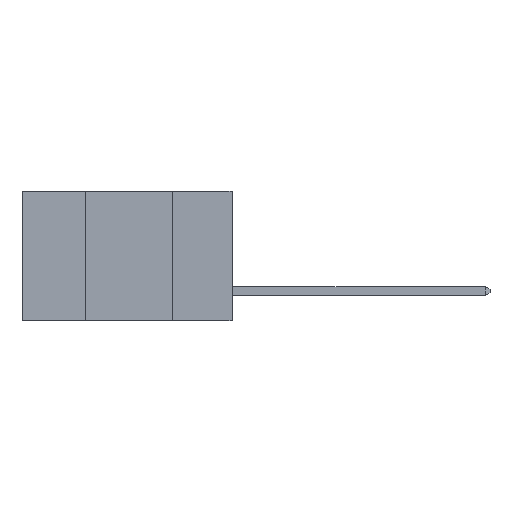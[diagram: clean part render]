
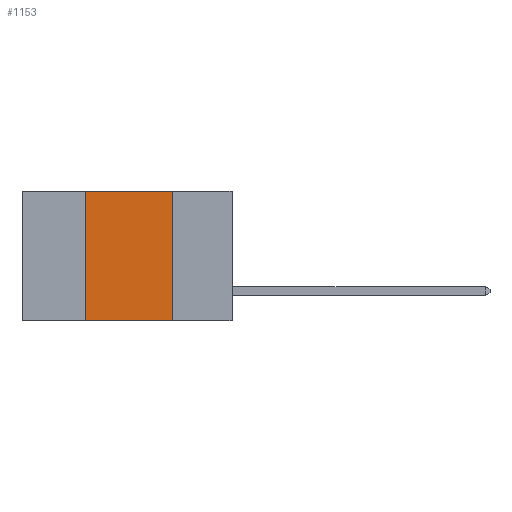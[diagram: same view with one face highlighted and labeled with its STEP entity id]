
A CAD part, left-side view. The second image highlights one B-rep face of the part: STEP entity #1153.
In plain terms, the highlighted planar face has unit normal (-1, 0, 0).
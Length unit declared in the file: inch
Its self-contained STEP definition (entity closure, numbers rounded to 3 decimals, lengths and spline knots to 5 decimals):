
#1010 = CARTESIAN_POINT ( 'NONE',  ( 0., 0.42, 0. ) ) ;
#1065 = EDGE_LOOP ( 'NONE', ( #1252, #15405, #2846, #11897 ) ) ;
#1153 = ADVANCED_FACE ( 'NONE', ( #24720 ), #20510, .F. ) ;
#1252 = ORIENTED_EDGE ( 'NONE', *, *, #6968, .F. ) ;
#2185 = CARTESIAN_POINT ( 'NONE',  ( 0., 0.6, -0.37 ) ) ;
#2846 = ORIENTED_EDGE ( 'NONE', *, *, #15335, .F. ) ;
#5372 = LINE ( 'NONE', #12961, #31651 ) ;
#6355 = VECTOR ( 'NONE', #9784, 39.37008 ) ;
#6968 = EDGE_CURVE ( 'NONE', #22509, #12967, #28034, .T. ) ;
#8129 = DIRECTION ( 'NONE',  ( 0., 0., -1. ) ) ;
#9151 = VECTOR ( 'NONE', #26149, 39.37008 ) ;
#9160 = EDGE_CURVE ( 'NONE', #28784, #12967, #13029, .T. ) ;
#9784 = DIRECTION ( 'NONE',  ( 0., -1., 0. ) ) ;
#10506 = CARTESIAN_POINT ( 'NONE',  ( 0., 0.6, 0. ) ) ;
#11268 = CARTESIAN_POINT ( 'NONE',  ( 0., 0.17, 0. ) ) ;
#11897 = ORIENTED_EDGE ( 'NONE', *, *, #9160, .T. ) ;
#12961 = CARTESIAN_POINT ( 'NONE',  ( 0., 0.42, 0. ) ) ;
#12967 = VERTEX_POINT ( 'NONE', #18007 ) ;
#13029 = LINE ( 'NONE', #2185, #6355 ) ;
#14390 = DIRECTION ( 'NONE',  ( 0., -1., 0. ) ) ;
#15335 = EDGE_CURVE ( 'NONE', #28784, #18723, #5372, .T. ) ;
#15405 = ORIENTED_EDGE ( 'NONE', *, *, #31181, .F. ) ;
#15458 = DIRECTION ( 'NONE',  ( 0., 0., 1. ) ) ;
#16100 = CARTESIAN_POINT ( 'NONE',  ( 0., 0.17, 0. ) ) ;
#18007 = CARTESIAN_POINT ( 'NONE',  ( 0., 0.17, -0.37 ) ) ;
#18699 = VECTOR ( 'NONE', #14390, 39.37008 ) ;
#18723 = VERTEX_POINT ( 'NONE', #1010 ) ;
#20510 = PLANE ( 'NONE',  #24918 ) ;
#21654 = CARTESIAN_POINT ( 'NONE',  ( 0., 0.42, -0.37 ) ) ;
#22509 = VERTEX_POINT ( 'NONE', #16100 ) ;
#22967 = DIRECTION ( 'NONE',  ( 1., 0., 0. ) ) ;
#24720 = FACE_OUTER_BOUND ( 'NONE', #1065, .T. ) ;
#24918 = AXIS2_PLACEMENT_3D ( 'NONE', #10506, #22967, #8129 ) ;
#25217 = LINE ( 'NONE', #31539, #18699 ) ;
#26149 = DIRECTION ( 'NONE',  ( 0., 0., -1. ) ) ;
#28034 = LINE ( 'NONE', #11268, #9151 ) ;
#28784 = VERTEX_POINT ( 'NONE', #21654 ) ;
#31181 = EDGE_CURVE ( 'NONE', #18723, #22509, #25217, .T. ) ;
#31539 = CARTESIAN_POINT ( 'NONE',  ( 0., 0.6, 0. ) ) ;
#31651 = VECTOR ( 'NONE', #15458, 39.37008 ) ;
